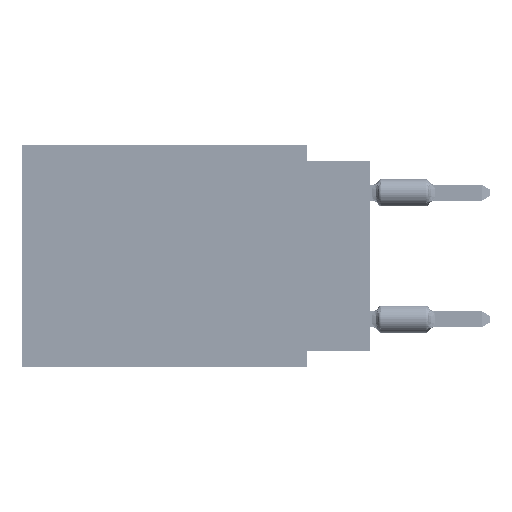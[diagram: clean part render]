
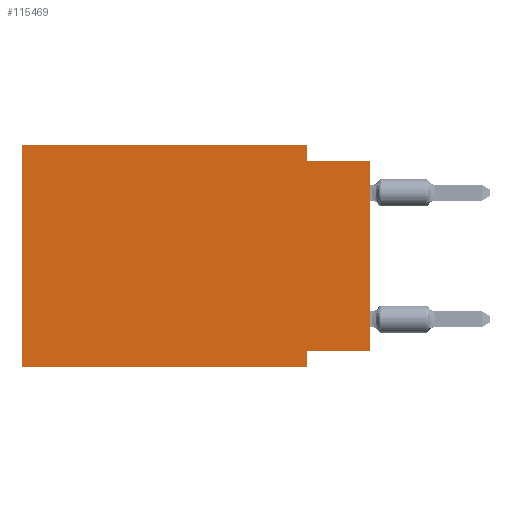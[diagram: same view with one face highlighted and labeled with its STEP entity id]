
A CAD part, left-side view. The second image highlights one B-rep face of the part: STEP entity #115469.
In plain terms, the highlighted planar face has unit normal (-1, 0, 0).
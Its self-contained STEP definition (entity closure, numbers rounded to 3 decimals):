
#4957 = CARTESIAN_POINT ( 'NONE',  ( 0., 13.97, -8.89 ) ) ;
#5188 = CARTESIAN_POINT ( 'NONE',  ( 0., 2.54, -8.89 ) ) ;
#6541 = DIRECTION ( 'NONE',  ( 0., -1., 0. ) ) ;
#9728 = EDGE_CURVE ( 'NONE', #60465, #114876, #20207, .T. ) ;
#9858 = ORIENTED_EDGE ( 'NONE', *, *, #76133, .F. ) ;
#9897 = EDGE_CURVE ( 'NONE', #60465, #107003, #33354, .T. ) ;
#11250 = VECTOR ( 'NONE', #40582, 1000. ) ;
#11741 = DIRECTION ( 'NONE',  ( 0., 0., 1. ) ) ;
#16997 = DIRECTION ( 'NONE',  ( 0., 0., 1. ) ) ;
#20207 = LINE ( 'NONE', #111059, #47723 ) ;
#20410 = DIRECTION ( 'NONE',  ( 0., -1., 0. ) ) ;
#21746 = EDGE_CURVE ( 'NONE', #71447, #90115, #76589, .T. ) ;
#22310 = CARTESIAN_POINT ( 'NONE',  ( 0., 0., -8.255 ) ) ;
#22686 = VERTEX_POINT ( 'NONE', #69843 ) ;
#25324 = ORIENTED_EDGE ( 'NONE', *, *, #40367, .F. ) ;
#26734 = ORIENTED_EDGE ( 'NONE', *, *, #21746, .T. ) ;
#30494 = AXIS2_PLACEMENT_3D ( 'NONE', #97393, #96200, #79957 ) ;
#31464 = VERTEX_POINT ( 'NONE', #104780 ) ;
#33354 = LINE ( 'NONE', #51386, #11250 ) ;
#33625 = PLANE ( 'NONE',  #30494 ) ;
#33660 = LINE ( 'NONE', #95080, #48717 ) ;
#34257 = ORIENTED_EDGE ( 'NONE', *, *, #9897, .F. ) ;
#38117 = VERTEX_POINT ( 'NONE', #116124 ) ;
#40367 = EDGE_CURVE ( 'NONE', #22686, #114876, #66127, .T. ) ;
#40582 = DIRECTION ( 'NONE',  ( 0., 1., 0. ) ) ;
#45115 = ORIENTED_EDGE ( 'NONE', *, *, #9728, .T. ) ;
#45861 = LINE ( 'NONE', #63922, #67863 ) ;
#46415 = VECTOR ( 'NONE', #16997, 1000. ) ;
#47588 = CARTESIAN_POINT ( 'NONE',  ( 0., 13.97, -8.89 ) ) ;
#47723 = VECTOR ( 'NONE', #11741, 1000. ) ;
#47813 = EDGE_CURVE ( 'NONE', #71447, #38117, #57686, .T. ) ;
#48717 = VECTOR ( 'NONE', #70351, 1000. ) ;
#50160 = CARTESIAN_POINT ( 'NONE',  ( 0., 2.54, -8.255 ) ) ;
#51386 = CARTESIAN_POINT ( 'NONE',  ( 0., 0., -8.255 ) ) ;
#57686 = LINE ( 'NONE', #91589, #46415 ) ;
#59105 = DIRECTION ( 'NONE',  ( 0., -1., 0. ) ) ;
#59610 = EDGE_CURVE ( 'NONE', #31464, #22686, #45861, .T. ) ;
#60465 = VERTEX_POINT ( 'NONE', #22310 ) ;
#63922 = CARTESIAN_POINT ( 'NONE',  ( 0., 2.54, 0. ) ) ;
#66127 = LINE ( 'NONE', #102836, #100612 ) ;
#67863 = VECTOR ( 'NONE', #82589, 1000. ) ;
#68628 = EDGE_CURVE ( 'NONE', #107003, #90115, #33660, .T. ) ;
#69843 = CARTESIAN_POINT ( 'NONE',  ( 0., 2.54, -0.635 ) ) ;
#70351 = DIRECTION ( 'NONE',  ( 0., 0., -1. ) ) ;
#70377 = VECTOR ( 'NONE', #59105, 1000. ) ;
#71447 = VERTEX_POINT ( 'NONE', #47588 ) ;
#72280 = ORIENTED_EDGE ( 'NONE', *, *, #47813, .F. ) ;
#76133 = EDGE_CURVE ( 'NONE', #38117, #31464, #97987, .T. ) ;
#76589 = LINE ( 'NONE', #4957, #70377 ) ;
#79592 = VECTOR ( 'NONE', #6541, 1000. ) ;
#79957 = DIRECTION ( 'NONE',  ( 0., 0., -1. ) ) ;
#82589 = DIRECTION ( 'NONE',  ( 0., 0., -1. ) ) ;
#89710 = ORIENTED_EDGE ( 'NONE', *, *, #59610, .F. ) ;
#90115 = VERTEX_POINT ( 'NONE', #5188 ) ;
#91589 = CARTESIAN_POINT ( 'NONE',  ( 0., 13.97, 0. ) ) ;
#95080 = CARTESIAN_POINT ( 'NONE',  ( 0., 2.54, -8.89 ) ) ;
#96200 = DIRECTION ( 'NONE',  ( 1., 0., 0. ) ) ;
#96208 = CARTESIAN_POINT ( 'NONE',  ( 0., 13.97, 0. ) ) ;
#97393 = CARTESIAN_POINT ( 'NONE',  ( 0., 13.97, 0. ) ) ;
#97987 = LINE ( 'NONE', #96208, #79592 ) ;
#100612 = VECTOR ( 'NONE', #20410, 1000. ) ;
#102836 = CARTESIAN_POINT ( 'NONE',  ( 0., 0., -0.635 ) ) ;
#104780 = CARTESIAN_POINT ( 'NONE',  ( 0., 2.54, 0. ) ) ;
#107003 = VERTEX_POINT ( 'NONE', #50160 ) ;
#107044 = ORIENTED_EDGE ( 'NONE', *, *, #68628, .F. ) ;
#110421 = CARTESIAN_POINT ( 'NONE',  ( 0., 0., -0.635 ) ) ;
#111059 = CARTESIAN_POINT ( 'NONE',  ( 0., 0., 0. ) ) ;
#113099 = EDGE_LOOP ( 'NONE', ( #45115, #25324, #89710, #9858, #72280, #26734, #107044, #34257 ) ) ;
#114876 = VERTEX_POINT ( 'NONE', #110421 ) ;
#115469 = ADVANCED_FACE ( 'NONE', ( #116046 ), #33625, .F. ) ;
#116046 = FACE_OUTER_BOUND ( 'NONE', #113099, .T. ) ;
#116124 = CARTESIAN_POINT ( 'NONE',  ( 0., 13.97, 0. ) ) ;
